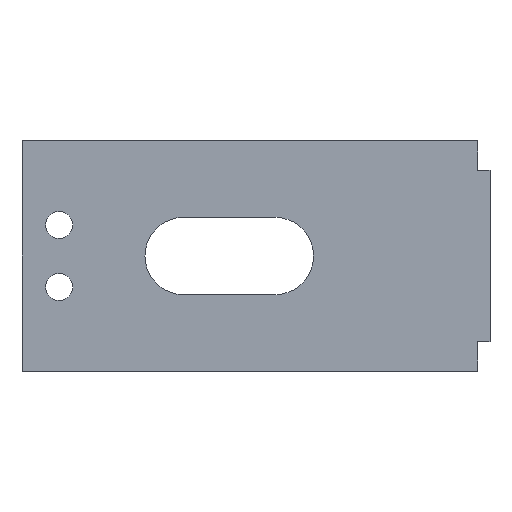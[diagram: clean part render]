
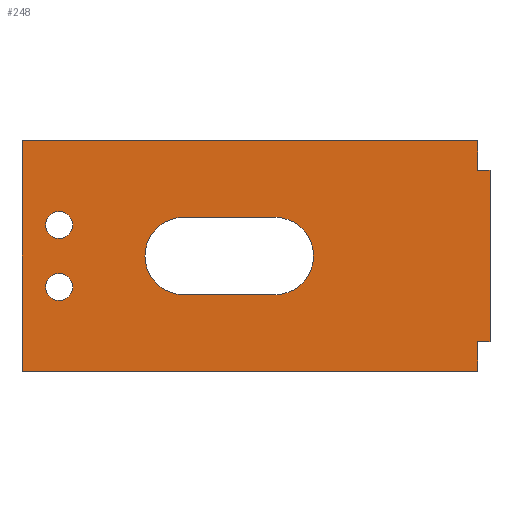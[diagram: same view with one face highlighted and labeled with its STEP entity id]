
A CAD part, front view. The second image highlights one B-rep face of the part: STEP entity #248.
In plain terms, the highlighted planar face has unit normal (0, -1, 0).
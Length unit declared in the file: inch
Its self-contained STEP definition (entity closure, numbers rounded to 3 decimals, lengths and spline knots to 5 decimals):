
#5 = CARTESIAN_POINT ( 'NONE',  ( 0.15, -0.125, -0.59 ) ) ;
#11 = VECTOR ( 'NONE', #12, 39.37008 ) ;
#12 = DIRECTION ( 'NONE',  ( 1., 0., 0. ) ) ;
#23 = CARTESIAN_POINT ( 'NONE',  ( 0., -0.125, -0.93 ) ) ;
#26 = FACE_BOUND ( 'NONE', #459, .T. ) ;
#35 = ORIENTED_EDGE ( 'NONE', *, *, #642, .T. ) ;
#38 = AXIS2_PLACEMENT_3D ( 'NONE', #149, #633, #220 ) ;
#46 = LINE ( 'NONE', #144, #11 ) ;
#58 = ORIENTED_EDGE ( 'NONE', *, *, #870, .T. ) ;
#62 = VECTOR ( 'NONE', #709, 39.37008 ) ;
#63 = EDGE_CURVE ( 'NONE', #354, #537, #345, .T. ) ;
#64 = ORIENTED_EDGE ( 'NONE', *, *, #842, .F. ) ;
#70 = CARTESIAN_POINT ( 'NONE',  ( 0.15, -0.125, -0.59 ) ) ;
#87 = CARTESIAN_POINT ( 'NONE',  ( 0.6523, -0.125, -0.465 ) ) ;
#90 = DIRECTION ( 'NONE',  ( 0., 0., 1. ) ) ;
#110 = VECTOR ( 'NONE', #697, 39.37008 ) ;
#136 = CARTESIAN_POINT ( 'NONE',  ( 1.888, -0.125, -0.81 ) ) ;
#142 = DIRECTION ( 'NONE',  ( 0., 0., 1. ) ) ;
#144 = CARTESIAN_POINT ( 'NONE',  ( 0., -0.125, 0. ) ) ;
#147 = VERTEX_POINT ( 'NONE', #403 ) ;
#149 = CARTESIAN_POINT ( 'NONE',  ( 0.15, -0.125, -0.34 ) ) ;
#158 = DIRECTION ( 'NONE',  ( 0., 0., 1. ) ) ;
#160 = CARTESIAN_POINT ( 'NONE',  ( 0., -0.125, 0. ) ) ;
#162 = EDGE_LOOP ( 'NONE', ( #58, #441, #35, #838 ) ) ;
#164 = CARTESIAN_POINT ( 'NONE',  ( 1.0198, -0.125, -0.3087 ) ) ;
#171 = VERTEX_POINT ( 'NONE', #400 ) ;
#181 = VECTOR ( 'NONE', #835, 39.37008 ) ;
#196 = EDGE_CURVE ( 'NONE', #414, #613, #448, .T. ) ;
#197 = EDGE_CURVE ( 'NONE', #871, #265, #253, .T. ) ;
#198 = EDGE_CURVE ( 'NONE', #387, #634, #505, .T. ) ;
#199 = LINE ( 'NONE', #445, #350 ) ;
#206 = FACE_BOUND ( 'NONE', #341, .T. ) ;
#208 = CARTESIAN_POINT ( 'NONE',  ( 0.15, -0.125, -0.34 ) ) ;
#219 = LINE ( 'NONE', #274, #760 ) ;
#220 = DIRECTION ( 'NONE',  ( 0., 0., 1. ) ) ;
#223 = CARTESIAN_POINT ( 'NONE',  ( 1.0198, -0.125, -0.6213 ) ) ;
#224 = PLANE ( 'NONE',  #470 ) ;
#231 = VECTOR ( 'NONE', #639, 39.37008 ) ;
#248 = ADVANCED_FACE ( 'NONE', ( #423, #751, #26, #206 ), #224, .F. ) ;
#249 = ORIENTED_EDGE ( 'NONE', *, *, #198, .T. ) ;
#253 = LINE ( 'NONE', #774, #595 ) ;
#255 = LINE ( 'NONE', #556, #733 ) ;
#258 = VERTEX_POINT ( 'NONE', #23 ) ;
#259 = AXIS2_PLACEMENT_3D ( 'NONE', #70, #555, #142 ) ;
#265 = VERTEX_POINT ( 'NONE', #164 ) ;
#267 = CARTESIAN_POINT ( 'NONE',  ( 0.6523, -0.125, -0.6213 ) ) ;
#274 = CARTESIAN_POINT ( 'NONE',  ( 0., -0.125, -0.12 ) ) ;
#286 = DIRECTION ( 'NONE',  ( 0., 0., 1. ) ) ;
#299 = ORIENTED_EDGE ( 'NONE', *, *, #534, .T. ) ;
#318 = VECTOR ( 'NONE', #793, 39.37008 ) ;
#320 = ORIENTED_EDGE ( 'NONE', *, *, #63, .T. ) ;
#341 = EDGE_LOOP ( 'NONE', ( #320, #299 ) ) ;
#345 = CIRCLE ( 'NONE', #797, 0.0547 ) ;
#346 = EDGE_CURVE ( 'NONE', #561, #784, #692, .T. ) ;
#350 = VECTOR ( 'NONE', #506, 39.37008 ) ;
#354 = VERTEX_POINT ( 'NONE', #591 ) ;
#359 = CARTESIAN_POINT ( 'NONE',  ( 0.15, -0.125, -0.6447 ) ) ;
#366 = CARTESIAN_POINT ( 'NONE',  ( 1.838, -0.125, -0.81 ) ) ;
#368 = CIRCLE ( 'NONE', #837, 0.1563 ) ;
#371 = CARTESIAN_POINT ( 'NONE',  ( 1.0198, -0.125, -0.465 ) ) ;
#375 = DIRECTION ( 'NONE',  ( 0., 1., 0. ) ) ;
#387 = VERTEX_POINT ( 'NONE', #457 ) ;
#400 = CARTESIAN_POINT ( 'NONE',  ( 0., -0.125, 0. ) ) ;
#403 = CARTESIAN_POINT ( 'NONE',  ( 0.15, -0.125, -0.3947 ) ) ;
#405 = ORIENTED_EDGE ( 'NONE', *, *, #862, .T. ) ;
#414 = VERTEX_POINT ( 'NONE', #267 ) ;
#419 = ORIENTED_EDGE ( 'NONE', *, *, #572, .T. ) ;
#423 = FACE_OUTER_BOUND ( 'NONE', #517, .T. ) ;
#438 = DIRECTION ( 'NONE',  ( 0., 0., 1. ) ) ;
#441 = ORIENTED_EDGE ( 'NONE', *, *, #196, .F. ) ;
#445 = CARTESIAN_POINT ( 'NONE',  ( 1.838, -0.125, 0. ) ) ;
#448 = LINE ( 'NONE', #769, #62 ) ;
#457 = CARTESIAN_POINT ( 'NONE',  ( 1.838, -0.125, -0.12 ) ) ;
#459 = EDGE_LOOP ( 'NONE', ( #852, #405 ) ) ;
#462 = ORIENTED_EDGE ( 'NONE', *, *, #467, .F. ) ;
#463 = ORIENTED_EDGE ( 'NONE', *, *, #346, .T. ) ;
#467 = EDGE_CURVE ( 'NONE', #387, #593, #219, .T. ) ;
#470 = AXIS2_PLACEMENT_3D ( 'NONE', #160, #375, #90 ) ;
#500 = VERTEX_POINT ( 'NONE', #682 ) ;
#503 = CARTESIAN_POINT ( 'NONE',  ( 1.888, -0.125, 0. ) ) ;
#504 = LINE ( 'NONE', #627, #110 ) ;
#505 = LINE ( 'NONE', #508, #231 ) ;
#506 = DIRECTION ( 'NONE',  ( 0., 0., 1. ) ) ;
#508 = CARTESIAN_POINT ( 'NONE',  ( 1.838, -0.125, 0. ) ) ;
#517 = EDGE_LOOP ( 'NONE', ( #693, #463, #575, #462, #249, #64, #587, #419 ) ) ;
#521 = AXIS2_PLACEMENT_3D ( 'NONE', #208, #690, #286 ) ;
#525 = CARTESIAN_POINT ( 'NONE',  ( 0., -0.125, -0.81 ) ) ;
#534 = EDGE_CURVE ( 'NONE', #537, #354, #857, .T. ) ;
#537 = VERTEX_POINT ( 'NONE', #359 ) ;
#545 = DIRECTION ( 'NONE',  ( 0., 1., 0. ) ) ;
#546 = LINE ( 'NONE', #503, #181 ) ;
#555 = DIRECTION ( 'NONE',  ( 0., 1., 0. ) ) ;
#556 = CARTESIAN_POINT ( 'NONE',  ( 0., -0.125, 0. ) ) ;
#557 = CIRCLE ( 'NONE', #38, 0.0547 ) ;
#561 = VERTEX_POINT ( 'NONE', #366 ) ;
#563 = CARTESIAN_POINT ( 'NONE',  ( 0.6523, -0.125, -0.3087 ) ) ;
#572 = EDGE_CURVE ( 'NONE', #258, #714, #504, .T. ) ;
#573 = DIRECTION ( 'NONE',  ( 0., 1., 0. ) ) ;
#575 = ORIENTED_EDGE ( 'NONE', *, *, #616, .F. ) ;
#587 = ORIENTED_EDGE ( 'NONE', *, *, #828, .T. ) ;
#591 = CARTESIAN_POINT ( 'NONE',  ( 0.15, -0.125, -0.5353 ) ) ;
#593 = VERTEX_POINT ( 'NONE', #829 ) ;
#595 = VECTOR ( 'NONE', #707, 39.37008 ) ;
#600 = CIRCLE ( 'NONE', #521, 0.0547 ) ;
#613 = VERTEX_POINT ( 'NONE', #223 ) ;
#616 = EDGE_CURVE ( 'NONE', #593, #784, #546, .T. ) ;
#626 = DIRECTION ( 'NONE',  ( 0., 0., -1. ) ) ;
#627 = CARTESIAN_POINT ( 'NONE',  ( 0., -0.125, -0.93 ) ) ;
#633 = DIRECTION ( 'NONE',  ( 0., 1., 0. ) ) ;
#634 = VERTEX_POINT ( 'NONE', #771 ) ;
#639 = DIRECTION ( 'NONE',  ( 0., 0., 1. ) ) ;
#642 = EDGE_CURVE ( 'NONE', #414, #871, #880, .T. ) ;
#649 = CARTESIAN_POINT ( 'NONE',  ( 1.838, -0.125, -0.93 ) ) ;
#654 = EDGE_CURVE ( 'NONE', #714, #561, #199, .T. ) ;
#678 = DIRECTION ( 'NONE',  ( 1., 0., 0. ) ) ;
#682 = CARTESIAN_POINT ( 'NONE',  ( 0.15, -0.125, -0.2853 ) ) ;
#690 = DIRECTION ( 'NONE',  ( 0., 1., 0. ) ) ;
#692 = LINE ( 'NONE', #525, #318 ) ;
#693 = ORIENTED_EDGE ( 'NONE', *, *, #654, .T. ) ;
#697 = DIRECTION ( 'NONE',  ( 1., 0., 0. ) ) ;
#707 = DIRECTION ( 'NONE',  ( 1., 0., 0. ) ) ;
#709 = DIRECTION ( 'NONE',  ( 1., 0., 0. ) ) ;
#714 = VERTEX_POINT ( 'NONE', #649 ) ;
#733 = VECTOR ( 'NONE', #626, 39.37008 ) ;
#751 = FACE_BOUND ( 'NONE', #162, .T. ) ;
#759 = AXIS2_PLACEMENT_3D ( 'NONE', #87, #573, #158 ) ;
#760 = VECTOR ( 'NONE', #678, 39.37008 ) ;
#769 = CARTESIAN_POINT ( 'NONE',  ( 0., -0.125, -0.6213 ) ) ;
#771 = CARTESIAN_POINT ( 'NONE',  ( 1.838, -0.125, 0. ) ) ;
#774 = CARTESIAN_POINT ( 'NONE',  ( 0., -0.125, -0.3087 ) ) ;
#784 = VERTEX_POINT ( 'NONE', #136 ) ;
#793 = DIRECTION ( 'NONE',  ( 1., 0., 0. ) ) ;
#795 = EDGE_CURVE ( 'NONE', #500, #147, #600, .T. ) ;
#797 = AXIS2_PLACEMENT_3D ( 'NONE', #5, #545, #856 ) ;
#828 = EDGE_CURVE ( 'NONE', #171, #258, #255, .T. ) ;
#829 = CARTESIAN_POINT ( 'NONE',  ( 1.888, -0.125, -0.12 ) ) ;
#833 = DIRECTION ( 'NONE',  ( 0., 1., 0. ) ) ;
#835 = DIRECTION ( 'NONE',  ( 0., 0., -1. ) ) ;
#837 = AXIS2_PLACEMENT_3D ( 'NONE', #371, #833, #438 ) ;
#838 = ORIENTED_EDGE ( 'NONE', *, *, #197, .T. ) ;
#842 = EDGE_CURVE ( 'NONE', #171, #634, #46, .T. ) ;
#852 = ORIENTED_EDGE ( 'NONE', *, *, #795, .T. ) ;
#856 = DIRECTION ( 'NONE',  ( 0., 0., 1. ) ) ;
#857 = CIRCLE ( 'NONE', #259, 0.0547 ) ;
#862 = EDGE_CURVE ( 'NONE', #147, #500, #557, .T. ) ;
#870 = EDGE_CURVE ( 'NONE', #265, #613, #368, .T. ) ;
#871 = VERTEX_POINT ( 'NONE', #563 ) ;
#880 = CIRCLE ( 'NONE', #759, 0.1563 ) ;
